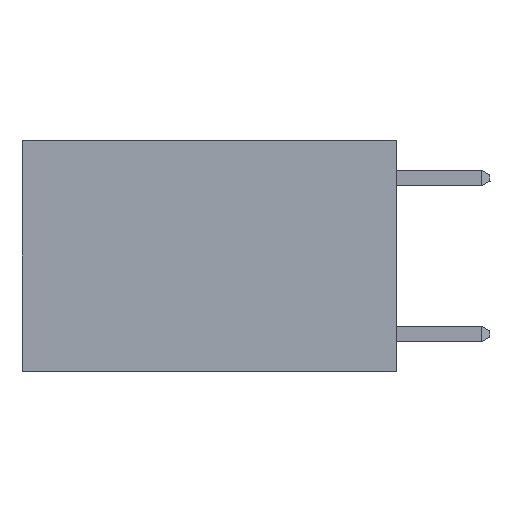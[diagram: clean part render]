
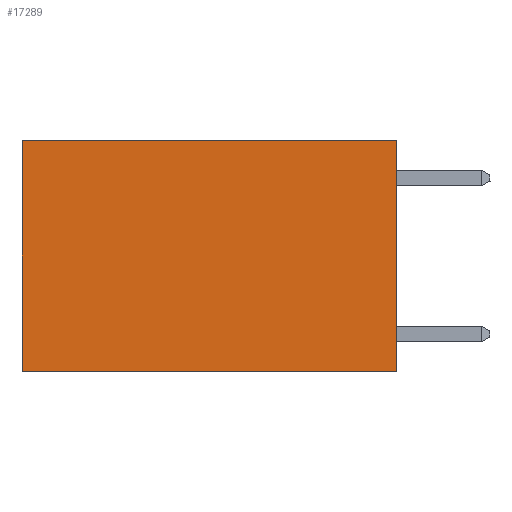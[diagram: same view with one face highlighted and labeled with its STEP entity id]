
A CAD part, left-side view. The second image highlights one B-rep face of the part: STEP entity #17289.
In plain terms, the highlighted planar face has unit normal (-1, 0, 0).
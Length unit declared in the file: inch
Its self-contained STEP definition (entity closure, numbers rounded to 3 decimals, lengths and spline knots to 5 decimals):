
#809 = DIRECTION ( 'NONE',  ( 1., 0., 0. ) ) ;
#1576 = VERTEX_POINT ( 'NONE', #5644 ) ;
#5644 = CARTESIAN_POINT ( 'NONE',  ( 0.2625, 0.6, 0. ) ) ;
#5853 = EDGE_CURVE ( 'NONE', #16646, #19882, #6707, .T. ) ;
#6315 = EDGE_CURVE ( 'NONE', #12865, #1576, #10887, .T. ) ;
#6689 = ORIENTED_EDGE ( 'NONE', *, *, #6315, .T. ) ;
#6707 = LINE ( 'NONE', #21884, #22501 ) ;
#6942 = CARTESIAN_POINT ( 'NONE',  ( 0.2625, 0., -0.37 ) ) ;
#8897 = AXIS2_PLACEMENT_3D ( 'NONE', #17518, #809, #15198 ) ;
#9987 = ORIENTED_EDGE ( 'NONE', *, *, #11144, .T. ) ;
#10549 = CARTESIAN_POINT ( 'NONE',  ( 0.2625, 0.6, 0. ) ) ;
#10639 = DIRECTION ( 'NONE',  ( 0., 0., -1. ) ) ;
#10887 = LINE ( 'NONE', #14917, #20537 ) ;
#11144 = EDGE_CURVE ( 'NONE', #1576, #19882, #26193, .T. ) ;
#12865 = VERTEX_POINT ( 'NONE', #17837 ) ;
#14710 = VECTOR ( 'NONE', #15898, 39.37008 ) ;
#14905 = VECTOR ( 'NONE', #10639, 39.37008 ) ;
#14917 = CARTESIAN_POINT ( 'NONE',  ( 0.2625, 0., 0. ) ) ;
#15198 = DIRECTION ( 'NONE',  ( 0., 0., -1. ) ) ;
#15898 = DIRECTION ( 'NONE',  ( 0., 0., -1. ) ) ;
#16646 = VERTEX_POINT ( 'NONE', #6942 ) ;
#16648 = LINE ( 'NONE', #26020, #14710 ) ;
#17221 = EDGE_LOOP ( 'NONE', ( #9987, #22947, #24074, #6689 ) ) ;
#17289 = ADVANCED_FACE ( 'NONE', ( #22612 ), #25486, .F. ) ;
#17518 = CARTESIAN_POINT ( 'NONE',  ( 0.2625, 0., 0. ) ) ;
#17837 = CARTESIAN_POINT ( 'NONE',  ( 0.2625, 0., 0. ) ) ;
#18547 = CARTESIAN_POINT ( 'NONE',  ( 0.2625, 0.6, -0.37 ) ) ;
#19882 = VERTEX_POINT ( 'NONE', #18547 ) ;
#20066 = DIRECTION ( 'NONE',  ( 0., 1., 0. ) ) ;
#20405 = EDGE_CURVE ( 'NONE', #12865, #16646, #16648, .T. ) ;
#20537 = VECTOR ( 'NONE', #23205, 39.37008 ) ;
#21884 = CARTESIAN_POINT ( 'NONE',  ( 0.2625, 0., -0.37 ) ) ;
#22501 = VECTOR ( 'NONE', #20066, 39.37008 ) ;
#22612 = FACE_OUTER_BOUND ( 'NONE', #17221, .T. ) ;
#22947 = ORIENTED_EDGE ( 'NONE', *, *, #5853, .F. ) ;
#23205 = DIRECTION ( 'NONE',  ( 0., 1., 0. ) ) ;
#24074 = ORIENTED_EDGE ( 'NONE', *, *, #20405, .F. ) ;
#25486 = PLANE ( 'NONE',  #8897 ) ;
#26020 = CARTESIAN_POINT ( 'NONE',  ( 0.2625, 0., 0. ) ) ;
#26193 = LINE ( 'NONE', #10549, #14905 ) ;
